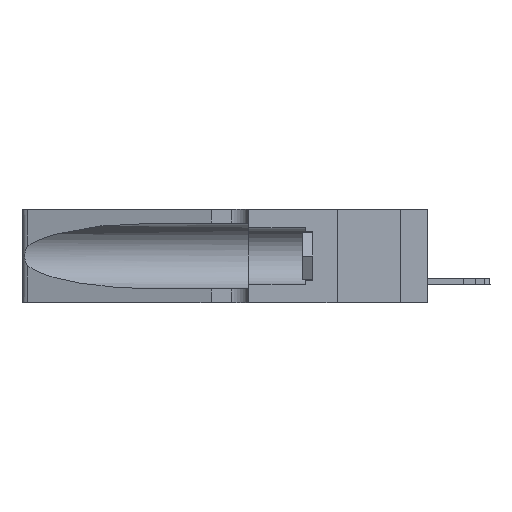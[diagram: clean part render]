
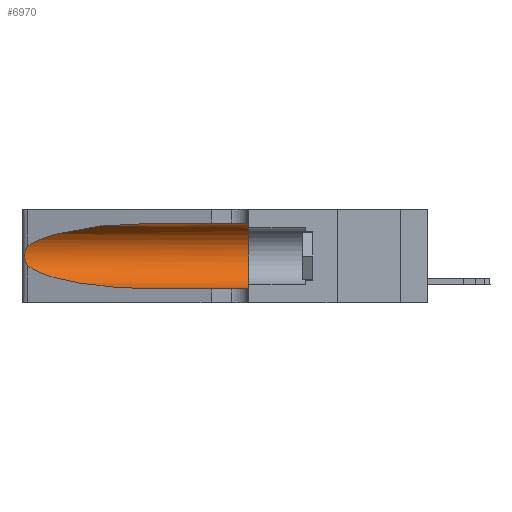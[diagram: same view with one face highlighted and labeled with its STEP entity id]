
A CAD part, left-side view. The second image highlights one B-rep face of the part: STEP entity #6970.
In plain terms, the highlighted cylindrical face has radius 3.308 mm (diameter 6.617 mm), a partial arc.
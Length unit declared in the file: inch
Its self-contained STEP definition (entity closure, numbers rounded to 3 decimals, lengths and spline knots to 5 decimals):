
#402 = DIRECTION ( 'NONE',  ( 0., -1., 0. ) ) ;
#417 = CARTESIAN_POINT ( 'NONE',  ( 0.26017, 1.23833, 0.17102 ) ) ;
#511 = CARTESIAN_POINT ( 'NONE',  ( 0.26075, 1.23896, 0.178 ) ) ;
#635 = CARTESIAN_POINT ( 'NONE',  ( 0.1305, 0.35, 0.05475 ) ) ;
#853 = EDGE_CURVE ( 'NONE', #7326, #15713, #21943, .T. ) ;
#1756 = ORIENTED_EDGE ( 'NONE', *, *, #7557, .F. ) ;
#2438 = ORIENTED_EDGE ( 'NONE', *, *, #22653, .T. ) ;
#2696 = AXIS2_PLACEMENT_3D ( 'NONE', #7737, #21411, #17614 ) ;
#3412 = CARTESIAN_POINT ( 'NONE',  ( 0.2373, 1.15595, 0.28018 ) ) ;
#3585 = ORIENTED_EDGE ( 'NONE', *, *, #853, .T. ) ;
#4660 = CARTESIAN_POINT ( 'NONE',  ( 0.25639, 1.23184, 0.21858 ) ) ;
#5046 = VECTOR ( 'NONE', #22831, 39.37008 ) ;
#5334 = AXIS2_PLACEMENT_3D ( 'NONE', #25036, #13101, #8814 ) ;
#5391 = CARTESIAN_POINT ( 'NONE',  ( 0.25487, 1.22718, 0.22369 ) ) ;
#5743 = ORIENTED_EDGE ( 'NONE', *, *, #16189, .T. ) ;
#6359 = VECTOR ( 'NONE', #402, 39.37008 ) ;
#6970 = ADVANCED_FACE ( 'NONE', ( #14001 ), #23974, .F. ) ;
#7326 = VERTEX_POINT ( 'NONE', #23481 ) ;
#7557 = EDGE_CURVE ( 'NONE', #14799, #22715, #17093, .T. ) ;
#7737 = CARTESIAN_POINT ( 'NONE',  ( 0.1305, 1.61858, 0.185 ) ) ;
#7972 = EDGE_LOOP ( 'NONE', ( #3585, #8413, #5743, #2438, #1756, #9510 ) ) ;
#8413 = ORIENTED_EDGE ( 'NONE', *, *, #13007, .T. ) ;
#8622 = EDGE_CURVE ( 'NONE', #7326, #14799, #17863, .T. ) ;
#8814 = DIRECTION ( 'NONE',  ( 0., 0., 1. ) ) ;
#9510 = ORIENTED_EDGE ( 'NONE', *, *, #8622, .F. ) ;
#10412 = CARTESIAN_POINT ( 'NONE',  ( 0.25555, 1.22994, 0.2215 ) ) ;
#10605 = CARTESIAN_POINT ( 'NONE',  ( 0.25487, 1.22718, 0.22369 ) ) ;
#12351 = CARTESIAN_POINT ( 'NONE',  ( 0.1305, 0.35, 0.31525 ) ) ;
#12399 = CARTESIAN_POINT ( 'NONE',  ( 0.25854, 1.2359, 0.20912 ) ) ;
#12586 = CARTESIAN_POINT ( 'NONE',  ( 0.26075, 1.23896, 0.19203 ) ) ;
#13007 = EDGE_CURVE ( 'NONE', #15713, #17783, #23858, .T. ) ;
#13101 = DIRECTION ( 'NONE',  ( 0., 1., 0. ) ) ;
#13467 = CARTESIAN_POINT ( 'NONE',  ( 0.18966, 0.96281, 0.05475 ) ) ;
#14001 = FACE_OUTER_BOUND ( 'NONE', #7972, .T. ) ;
#14403 = CARTESIAN_POINT ( 'NONE',  ( 0.25856, 1.23593, 0.16098 ) ) ;
#14579 = VERTEX_POINT ( 'NONE', #22564 ) ;
#14799 = VERTEX_POINT ( 'NONE', #12351 ) ;
#15205 = CARTESIAN_POINT ( 'NONE',  ( 0.1305, 0.72297, 0.05475 ) ) ;
#15713 = VERTEX_POINT ( 'NONE', #22132 ) ;
#16189 = EDGE_CURVE ( 'NONE', #17783, #14579, #25450, .T. ) ;
#16283 = CARTESIAN_POINT ( 'NONE',  ( 0.25555, 1.22993, 0.14849 ) ) ;
#16388 = CARTESIAN_POINT ( 'NONE',  ( 0.25789, 1.23486, 0.15765 ) ) ;
#16752 = CARTESIAN_POINT ( 'NONE',  ( 0.25487, 1.22718, 0.14631 ) ) ;
#17071 = CARTESIAN_POINT ( 'NONE',  ( 0.25487, 1.22718, 0.14631 ) ) ;
#17093 = CIRCLE ( 'NONE', #5334, 0.13025 ) ;
#17446 = CARTESIAN_POINT ( 'NONE',  ( 0.18966, 0.96281, 0.31525 ) ) ;
#17614 = DIRECTION ( 'NONE',  ( 0., 0., -1. ) ) ;
#17783 = VERTEX_POINT ( 'NONE', #16752 ) ;
#17863 = LINE ( 'NONE', #22234, #6359 ) ;
#18469 = CARTESIAN_POINT ( 'NONE',  ( 0.25487, 1.22718, 0.14631 ) ) ;
#18558 = CARTESIAN_POINT ( 'NONE',  ( 0.25639, 1.23186, 0.15144 ) ) ;
#18684 = CARTESIAN_POINT ( 'NONE',  ( 0.1305, 1.61858, 0.05475 ) ) ;
#19976 = LINE ( 'NONE', #18684, #5046 ) ;
#21411 = DIRECTION ( 'NONE',  ( 0., -1., 0. ) ) ;
#21943 =( BOUNDED_CURVE ( )  B_SPLINE_CURVE ( 3, ( #23343, #17446, #3412, #5391 ),
 .UNSPECIFIED., .F., .F. ) 
 B_SPLINE_CURVE_WITH_KNOTS ( ( 4, 4 ),
 ( 1.5708, 2.84003 ),
 .UNSPECIFIED. ) 
 CURVE ( )  GEOMETRIC_REPRESENTATION_ITEM ( )  RATIONAL_B_SPLINE_CURVE ( ( 1., 0.87, 0.87, 1. ) ) 
 REPRESENTATION_ITEM ( '' )  );
#22132 = CARTESIAN_POINT ( 'NONE',  ( 0.25487, 1.22718, 0.22369 ) ) ;
#22234 = CARTESIAN_POINT ( 'NONE',  ( 0.1305, 1.61858, 0.31525 ) ) ;
#22564 = CARTESIAN_POINT ( 'NONE',  ( 0.1305, 0.72297, 0.05475 ) ) ;
#22616 = CARTESIAN_POINT ( 'NONE',  ( 0.26018, 1.23835, 0.19895 ) ) ;
#22653 = EDGE_CURVE ( 'NONE', #14579, #22715, #19976, .T. ) ;
#22715 = VERTEX_POINT ( 'NONE', #635 ) ;
#22831 = DIRECTION ( 'NONE',  ( 0., -1., 0. ) ) ;
#23343 = CARTESIAN_POINT ( 'NONE',  ( 0.1305, 0.72297, 0.31525 ) ) ;
#23481 = CARTESIAN_POINT ( 'NONE',  ( 0.1305, 0.72297, 0.31525 ) ) ;
#23858 = B_SPLINE_CURVE_WITH_KNOTS ( 'NONE', 3,
 ( #10605, #10412, #4660, #24530, #12399, #22616, #12586, #511, #417, #14403, #16388, #18558, #16283, #18469 ),
 .UNSPECIFIED., .F., .F.,
 ( 4, 2, 2, 2, 2, 2, 4 ),
 ( 0., 0.00027, 0.00053, 0.00107, 0.0016, 0.00187, 0.00214 ),
 .UNSPECIFIED. ) ;
#23974 = CYLINDRICAL_SURFACE ( 'NONE', #2696, 0.13025 ) ;
#24530 = CARTESIAN_POINT ( 'NONE',  ( 0.25787, 1.23484, 0.2124 ) ) ;
#25036 = CARTESIAN_POINT ( 'NONE',  ( 0.1305, 0.35, 0.185 ) ) ;
#25240 = CARTESIAN_POINT ( 'NONE',  ( 0.2373, 1.15595, 0.08982 ) ) ;
#25450 =( BOUNDED_CURVE ( )  B_SPLINE_CURVE ( 3, ( #17071, #25240, #13467, #15205 ),
 .UNSPECIFIED., .F., .F. ) 
 B_SPLINE_CURVE_WITH_KNOTS ( ( 4, 4 ),
 ( 3.44316, 4.71239 ),
 .UNSPECIFIED. ) 
 CURVE ( )  GEOMETRIC_REPRESENTATION_ITEM ( )  RATIONAL_B_SPLINE_CURVE ( ( 1., 0.87, 0.87, 1. ) ) 
 REPRESENTATION_ITEM ( '' )  );
